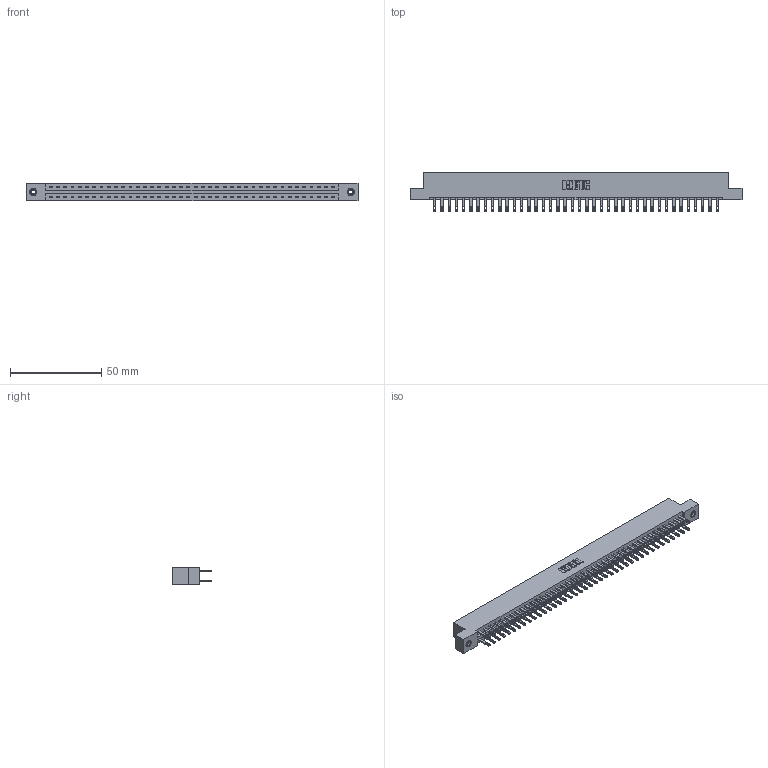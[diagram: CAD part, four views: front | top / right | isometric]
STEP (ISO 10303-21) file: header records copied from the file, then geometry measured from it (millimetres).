
FILE_DESCRIPTION (( 'STEP AP203' ), '1' );
FILE_NAME ('337-080-500-208.STEP', '2019-10-10T11:53:22', ( '' ), ( '' ), 'SwSTEP 2.0', 'SolidWorks 2016', '' );
FILE_SCHEMA (( 'CONFIG_CONTROL_DESIGN' ));
Length unit declared in the file: inch
Products named in the file (4): 345-292-001_345-293-100; 337 Part_Flush Mounting Lugs - 0.156 Dia-TI; 345-250-001_345-250-003-102; 337-080-500-208
Assembly tree (83 placements, depth 2):
  337-080-500-208
    337 Part_Flush Mounting Lugs - 0.156 Dia-TI
    345-292-001_345-293-100  x80
    345-250-001_345-250-003-102  x2
Bounding box: 181.51 x 21.85 x 9.4 mm (x, y, z)
Volume: 19340.1 mm3; surface area: 22756.2 mm2
Topology: 83 solids, 83 shells, 4174 faces, 12687 edges, 8450 vertices
Faces by surface type: plane 2662, cylinder 1496, cone 12, torus 4
Entity records: 32388 total; most frequent: CARTESIAN_POINT 5437, ORIENTED_EDGE 5366, DIRECTION 4661, EDGE_CURVE 2683, VECTOR 2531, LINE 2531, VERTEX_POINT 1784, AXIS2_PLACEMENT_3D 1065
